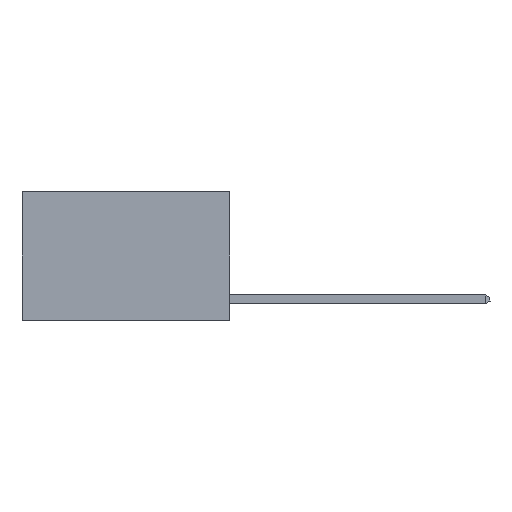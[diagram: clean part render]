
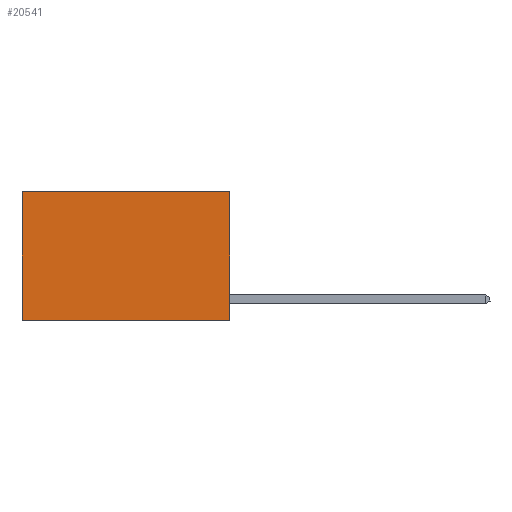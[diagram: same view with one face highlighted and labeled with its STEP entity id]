
A CAD part, left-side view. The second image highlights one B-rep face of the part: STEP entity #20541.
In plain terms, the highlighted planar face has unit normal (-1, 0, 0).
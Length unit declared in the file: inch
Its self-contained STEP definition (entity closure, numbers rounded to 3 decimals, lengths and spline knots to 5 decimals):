
#731 = LINE ( 'NONE', #17669, #4657 ) ;
#2862 = FACE_OUTER_BOUND ( 'NONE', #10854, .T. ) ;
#3066 = PLANE ( 'NONE',  #20371 ) ;
#3143 = DIRECTION ( 'NONE',  ( 0., 1., 0. ) ) ;
#4267 = DIRECTION ( 'NONE',  ( 0., 0., -1. ) ) ;
#4657 = VECTOR ( 'NONE', #20472, 39.37008 ) ;
#5849 = LINE ( 'NONE', #20690, #9574 ) ;
#5928 = LINE ( 'NONE', #12566, #17556 ) ;
#6122 = CARTESIAN_POINT ( 'NONE',  ( 0.2625, 0., 0. ) ) ;
#7512 = CARTESIAN_POINT ( 'NONE',  ( 0.2625, 0.6, -0.37 ) ) ;
#7803 = VERTEX_POINT ( 'NONE', #17968 ) ;
#9563 = ORIENTED_EDGE ( 'NONE', *, *, #16703, .F. ) ;
#9574 = VECTOR ( 'NONE', #10867, 39.37008 ) ;
#9750 = EDGE_CURVE ( 'NONE', #15781, #16783, #731, .T. ) ;
#10407 = ORIENTED_EDGE ( 'NONE', *, *, #10599, .T. ) ;
#10599 = EDGE_CURVE ( 'NONE', #16783, #17812, #5849, .T. ) ;
#10854 = EDGE_LOOP ( 'NONE', ( #10407, #9563, #11966, #14301 ) ) ;
#10867 = DIRECTION ( 'NONE',  ( 0., 0., -1. ) ) ;
#11099 = CARTESIAN_POINT ( 'NONE',  ( 0.2625, 0.6, 0. ) ) ;
#11966 = ORIENTED_EDGE ( 'NONE', *, *, #12063, .F. ) ;
#12063 = EDGE_CURVE ( 'NONE', #15781, #7803, #5928, .T. ) ;
#12566 = CARTESIAN_POINT ( 'NONE',  ( 0.2625, 0., 0. ) ) ;
#12949 = CARTESIAN_POINT ( 'NONE',  ( 0.2625, 0., -0.37 ) ) ;
#14301 = ORIENTED_EDGE ( 'NONE', *, *, #9750, .T. ) ;
#14372 = DIRECTION ( 'NONE',  ( 0., 0., -1. ) ) ;
#15781 = VERTEX_POINT ( 'NONE', #20973 ) ;
#16703 = EDGE_CURVE ( 'NONE', #7803, #17812, #21151, .T. ) ;
#16783 = VERTEX_POINT ( 'NONE', #11099 ) ;
#17556 = VECTOR ( 'NONE', #4267, 39.37008 ) ;
#17669 = CARTESIAN_POINT ( 'NONE',  ( 0.2625, 0., 0. ) ) ;
#17812 = VERTEX_POINT ( 'NONE', #7512 ) ;
#17968 = CARTESIAN_POINT ( 'NONE',  ( 0.2625, 0., -0.37 ) ) ;
#19406 = VECTOR ( 'NONE', #3143, 39.37008 ) ;
#20371 = AXIS2_PLACEMENT_3D ( 'NONE', #6122, #21187, #14372 ) ;
#20472 = DIRECTION ( 'NONE',  ( 0., 1., 0. ) ) ;
#20541 = ADVANCED_FACE ( 'NONE', ( #2862 ), #3066, .F. ) ;
#20690 = CARTESIAN_POINT ( 'NONE',  ( 0.2625, 0.6, 0. ) ) ;
#20973 = CARTESIAN_POINT ( 'NONE',  ( 0.2625, 0., 0. ) ) ;
#21151 = LINE ( 'NONE', #12949, #19406 ) ;
#21187 = DIRECTION ( 'NONE',  ( 1., 0., 0. ) ) ;
